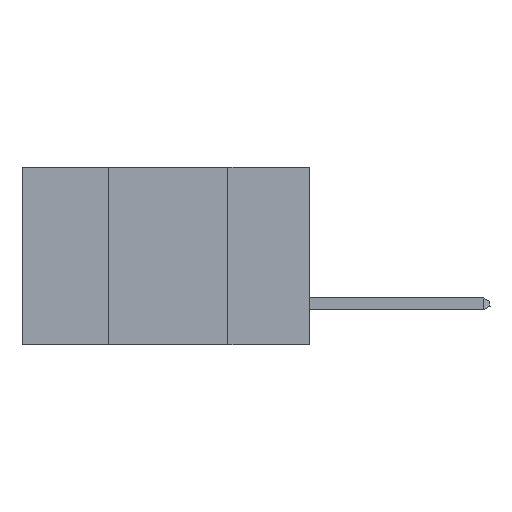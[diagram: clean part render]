
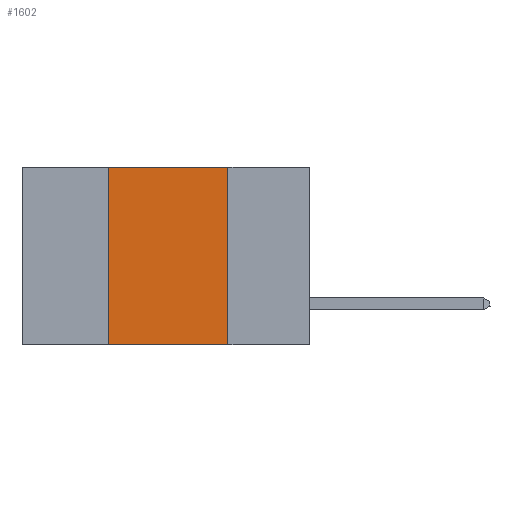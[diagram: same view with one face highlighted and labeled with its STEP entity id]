
A CAD part, left-side view. The second image highlights one B-rep face of the part: STEP entity #1602.
In plain terms, the highlighted planar face has unit normal (-1, 0, 0).
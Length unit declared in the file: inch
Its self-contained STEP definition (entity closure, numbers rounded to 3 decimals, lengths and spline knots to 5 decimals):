
#128 = VERTEX_POINT ( 'NONE', #831 ) ;
#168 = CARTESIAN_POINT ( 'NONE',  ( 0., 0.42, 0. ) ) ;
#260 = EDGE_CURVE ( 'NONE', #1646, #8816, #3479, .T. ) ;
#336 = EDGE_CURVE ( 'NONE', #1646, #2752, #8269, .T. ) ;
#831 = CARTESIAN_POINT ( 'NONE',  ( 0., 0.17, 0. ) ) ;
#909 = ORIENTED_EDGE ( 'NONE', *, *, #260, .F. ) ;
#1420 = CARTESIAN_POINT ( 'NONE',  ( 0., 0.42, -0.37 ) ) ;
#1602 = ADVANCED_FACE ( 'NONE', ( #5238 ), #6558, .F. ) ;
#1646 = VERTEX_POINT ( 'NONE', #1420 ) ;
#2307 = DIRECTION ( 'NONE',  ( 0., 0., 1. ) ) ;
#2426 = CARTESIAN_POINT ( 'NONE',  ( 0., 0.17, -0.37 ) ) ;
#2752 = VERTEX_POINT ( 'NONE', #2426 ) ;
#3409 = EDGE_CURVE ( 'NONE', #8816, #128, #4426, .T. ) ;
#3479 = LINE ( 'NONE', #7116, #3603 ) ;
#3495 = EDGE_LOOP ( 'NONE', ( #4651, #5485, #909, #6965 ) ) ;
#3603 = VECTOR ( 'NONE', #2307, 39.37008 ) ;
#3759 = DIRECTION ( 'NONE',  ( 0., 0., -1. ) ) ;
#4245 = DIRECTION ( 'NONE',  ( 0., 0., -1. ) ) ;
#4426 = LINE ( 'NONE', #7515, #7582 ) ;
#4651 = ORIENTED_EDGE ( 'NONE', *, *, #6776, .F. ) ;
#5202 = DIRECTION ( 'NONE',  ( 0., -1., 0. ) ) ;
#5238 = FACE_OUTER_BOUND ( 'NONE', #3495, .T. ) ;
#5485 = ORIENTED_EDGE ( 'NONE', *, *, #3409, .F. ) ;
#5841 = CARTESIAN_POINT ( 'NONE',  ( 0., 0.6, -0.37 ) ) ;
#6054 = DIRECTION ( 'NONE',  ( 0., -1., 0. ) ) ;
#6224 = VECTOR ( 'NONE', #5202, 39.37008 ) ;
#6393 = CARTESIAN_POINT ( 'NONE',  ( 0., 0.17, 0. ) ) ;
#6418 = LINE ( 'NONE', #6393, #6638 ) ;
#6558 = PLANE ( 'NONE',  #8093 ) ;
#6638 = VECTOR ( 'NONE', #4245, 39.37008 ) ;
#6776 = EDGE_CURVE ( 'NONE', #128, #2752, #6418, .T. ) ;
#6965 = ORIENTED_EDGE ( 'NONE', *, *, #336, .T. ) ;
#7116 = CARTESIAN_POINT ( 'NONE',  ( 0., 0.42, 0. ) ) ;
#7253 = CARTESIAN_POINT ( 'NONE',  ( 0., 0.6, 0. ) ) ;
#7515 = CARTESIAN_POINT ( 'NONE',  ( 0., 0.6, 0. ) ) ;
#7582 = VECTOR ( 'NONE', #6054, 39.37008 ) ;
#7933 = DIRECTION ( 'NONE',  ( 1., 0., 0. ) ) ;
#8093 = AXIS2_PLACEMENT_3D ( 'NONE', #7253, #7933, #3759 ) ;
#8269 = LINE ( 'NONE', #5841, #6224 ) ;
#8816 = VERTEX_POINT ( 'NONE', #168 ) ;
